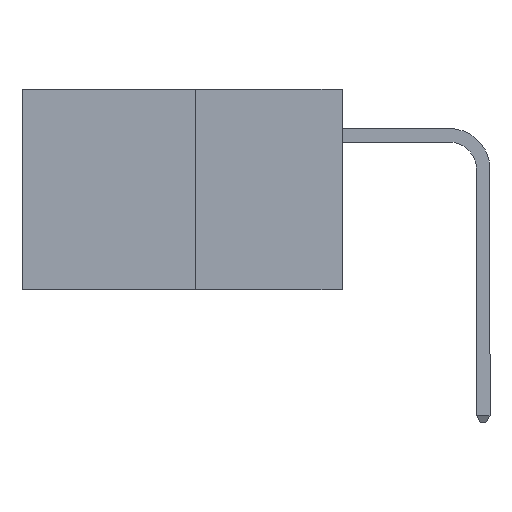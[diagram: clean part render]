
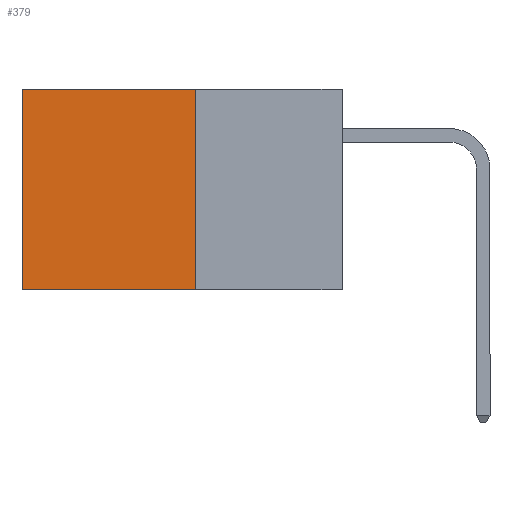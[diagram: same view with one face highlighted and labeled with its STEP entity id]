
A CAD part, left-side view. The second image highlights one B-rep face of the part: STEP entity #379.
In plain terms, the highlighted planar face has unit normal (-1, 0, 0).
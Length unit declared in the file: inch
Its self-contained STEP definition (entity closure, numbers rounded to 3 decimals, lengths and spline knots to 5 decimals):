
#294 = ORIENTED_EDGE ( 'NONE', *, *, #1206, .T. ) ;
#379 = ADVANCED_FACE ( 'NONE', ( #5582 ), #4520, .F. ) ;
#520 = EDGE_CURVE ( 'NONE', #3934, #9008, #4269, .T. ) ;
#736 = VERTEX_POINT ( 'NONE', #5110 ) ;
#756 = ORIENTED_EDGE ( 'NONE', *, *, #520, .F. ) ;
#842 = CARTESIAN_POINT ( 'NONE',  ( 0.277, 0.59, -0.37 ) ) ;
#926 = DIRECTION ( 'NONE',  ( 0., 1., 0. ) ) ;
#1122 = CARTESIAN_POINT ( 'NONE',  ( 0.277, 0.59, -0.37 ) ) ;
#1206 = EDGE_CURVE ( 'NONE', #736, #9008, #7090, .T. ) ;
#1924 = DIRECTION ( 'NONE',  ( 1., 0., 0. ) ) ;
#2033 = CARTESIAN_POINT ( 'NONE',  ( 0.277, 0.27, -0.37 ) ) ;
#3560 = EDGE_CURVE ( 'NONE', #6770, #736, #7681, .T. ) ;
#3883 = DIRECTION ( 'NONE',  ( 0., 1., 0. ) ) ;
#3934 = VERTEX_POINT ( 'NONE', #6801 ) ;
#4269 = LINE ( 'NONE', #2033, #8354 ) ;
#4274 = ORIENTED_EDGE ( 'NONE', *, *, #10233, .F. ) ;
#4310 = DIRECTION ( 'NONE',  ( 0., 0., -1. ) ) ;
#4520 = PLANE ( 'NONE',  #6421 ) ;
#4621 = DIRECTION ( 'NONE',  ( 0., 0., -1. ) ) ;
#4709 = CARTESIAN_POINT ( 'NONE',  ( 0.277, 0.27, -0.37 ) ) ;
#4787 = EDGE_LOOP ( 'NONE', ( #294, #756, #4274, #5102 ) ) ;
#5102 = ORIENTED_EDGE ( 'NONE', *, *, #3560, .T. ) ;
#5110 = CARTESIAN_POINT ( 'NONE',  ( 0.277, 0.59, 0. ) ) ;
#5519 = VECTOR ( 'NONE', #3883, 39.37008 ) ;
#5582 = FACE_OUTER_BOUND ( 'NONE', #4787, .T. ) ;
#5977 = CARTESIAN_POINT ( 'NONE',  ( 0.277, 0.27, 0. ) ) ;
#6421 = AXIS2_PLACEMENT_3D ( 'NONE', #4709, #1924, #6940 ) ;
#6567 = VECTOR ( 'NONE', #4621, 39.37008 ) ;
#6770 = VERTEX_POINT ( 'NONE', #5977 ) ;
#6801 = CARTESIAN_POINT ( 'NONE',  ( 0.277, 0.27, -0.37 ) ) ;
#6940 = DIRECTION ( 'NONE',  ( 0., 0., -1. ) ) ;
#7090 = LINE ( 'NONE', #1122, #6567 ) ;
#7681 = LINE ( 'NONE', #7924, #5519 ) ;
#7924 = CARTESIAN_POINT ( 'NONE',  ( 0.277, 0.27, 0. ) ) ;
#8354 = VECTOR ( 'NONE', #926, 39.37008 ) ;
#9008 = VERTEX_POINT ( 'NONE', #842 ) ;
#9882 = CARTESIAN_POINT ( 'NONE',  ( 0.277, 0.27, -0.37 ) ) ;
#9977 = VECTOR ( 'NONE', #4310, 39.37008 ) ;
#10210 = LINE ( 'NONE', #9882, #9977 ) ;
#10233 = EDGE_CURVE ( 'NONE', #6770, #3934, #10210, .T. ) ;
